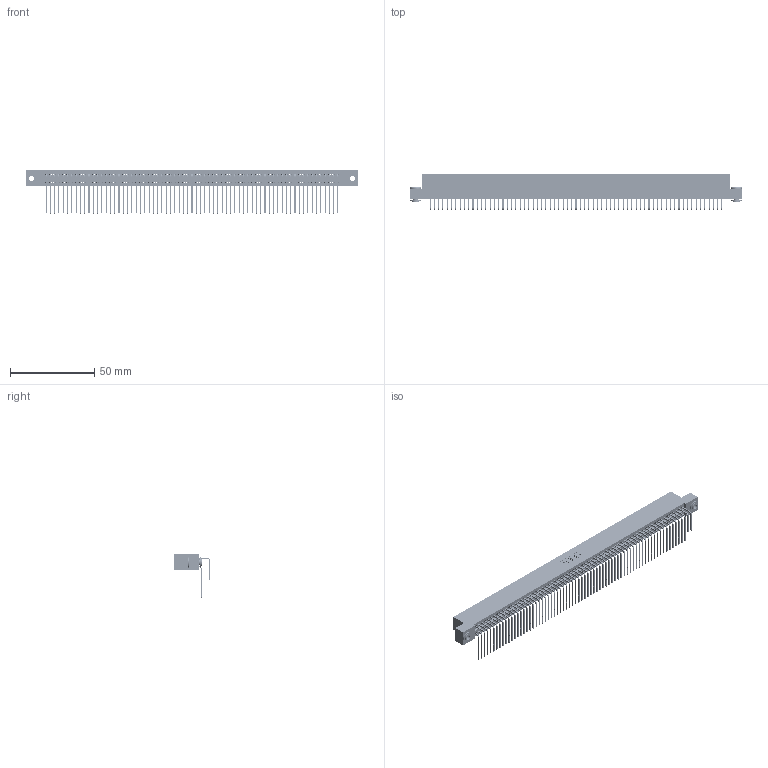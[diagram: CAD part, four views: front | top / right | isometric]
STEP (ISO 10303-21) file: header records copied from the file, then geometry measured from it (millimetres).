
FILE_DESCRIPTION (( 'STEP AP203' ), '1' );
FILE_NAME ('395-138-558-203.STEP', '2019-10-29T22:20:08', ( '' ), ( '' ), 'SwSTEP 2.0', 'SolidWorks 2016', '' );
FILE_SCHEMA (( 'CONFIG_CONTROL_DESIGN' ));
Length unit declared in the file: inch
Products named in the file (5): 345-292-001_558 559 Tail - 1; 345-292-001_558 Tail - 2; 345-250-002_345-250-002-102; 395-138-558-203; 345 Part_Flush Mounting Lugs - 0.156 Dia-TH
Assembly tree (141 placements, depth 2):
  395-138-558-203
    345 Part_Flush Mounting Lugs - 0.156 Dia-TH
    345-292-001_558 559 Tail - 1  x69
    345-292-001_558 Tail - 2  x69
    345-250-002_345-250-002-102  x2
Bounding box: 196.47 x 21.83 x 25.53 mm (x, y, z)
Volume: 20151.3 mm3; surface area: 34258.3 mm2
Topology: 141 solids, 141 shells, 7340 faces, 21807 edges, 14350 vertices
Faces by surface type: plane 4920, cylinder 2412, cone 8
Entity records: 52806 total; most frequent: CARTESIAN_POINT 8846, ORIENTED_EDGE 8722, DIRECTION 7771, EDGE_CURVE 4361, LINE 3889, VECTOR 3889, VERTEX_POINT 2902, AXIS2_PLACEMENT_3D 1941
